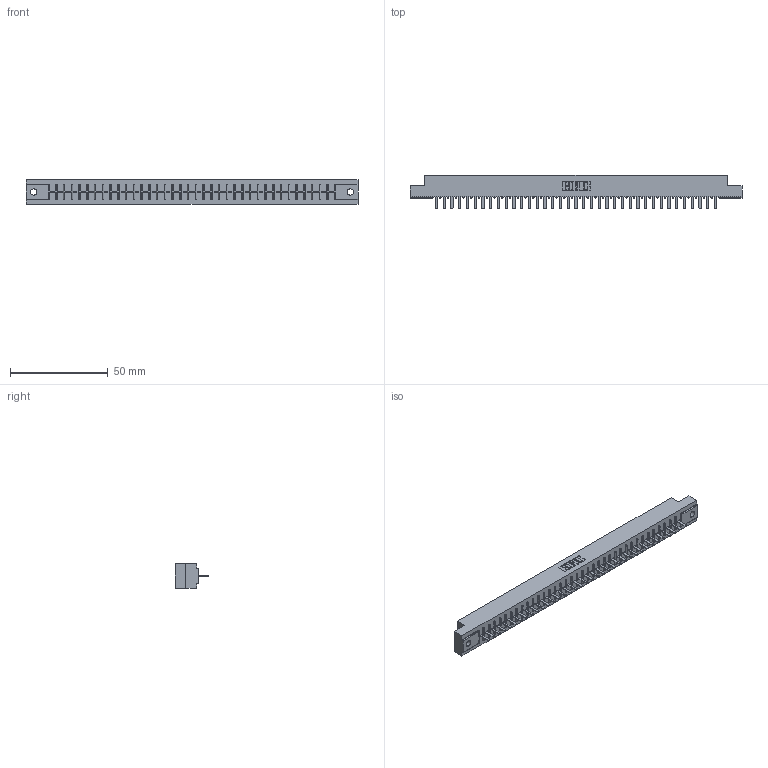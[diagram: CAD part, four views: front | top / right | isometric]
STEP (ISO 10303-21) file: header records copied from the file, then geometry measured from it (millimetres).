
FILE_DESCRIPTION (( 'STEP AP203' ), '1' );
FILE_NAME ('356-037-420-102.STEP', '2020-09-23T23:13:38', ( '' ), ( '' ), 'SwSTEP 2.0', 'SolidWorks 2020', '' );
FILE_SCHEMA (( 'CONFIG_CONTROL_DESIGN' ));
Length unit declared in the file: inch
Products named in the file (3): 306 Part_.128 Dia; 356-037-420-102; 306-290-001_120
Assembly tree (38 placements, depth 2):
  356-037-420-102
    306 Part_.128 Dia
    306-290-001_120  x37
Bounding box: 169.62 x 17.12 x 12.7 mm (x, y, z)
Volume: 18680.2 mm3; surface area: 18861.9 mm2
Topology: 38 solids, 38 shells, 2706 faces, 7605 edges, 4870 vertices
Faces by surface type: plane 1807, cylinder 751, sphere 148
Entity records: 35110 total; most frequent: CARTESIAN_POINT 5894, ORIENTED_EDGE 5842, DIRECTION 5813, EDGE_CURVE 2921, VECTOR 2283, LINE 2283, VERTEX_POINT 1846, AXIS2_PLACEMENT_3D 1765
